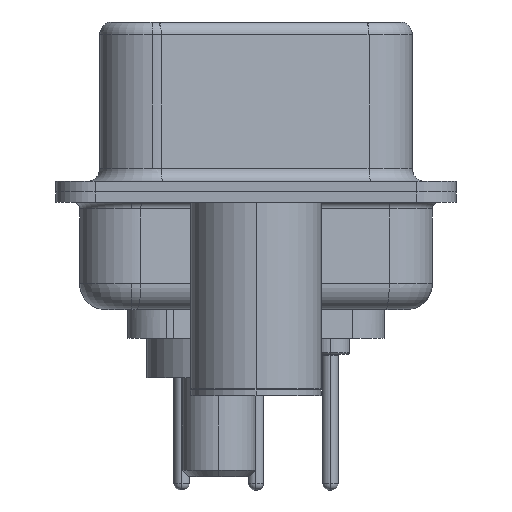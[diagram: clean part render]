
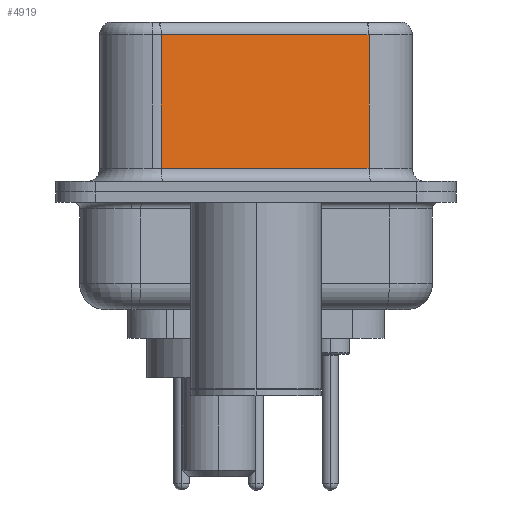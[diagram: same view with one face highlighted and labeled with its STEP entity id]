
A CAD part, left-side view. The second image highlights one B-rep face of the part: STEP entity #4919.
In plain terms, the highlighted planar face has unit normal (-0.985, -0.174, 0).
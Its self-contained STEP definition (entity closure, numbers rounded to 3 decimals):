
#663 = CARTESIAN_POINT ( 'NONE',  ( 5.132, -4.322, 6.52 ) ) ;
#1661 = ORIENTED_EDGE ( 'NONE', *, *, #18239, .T. ) ;
#2152 = CARTESIAN_POINT ( 'NONE',  ( 5.132, -4.322, 0.9 ) ) ;
#4515 = DIRECTION ( 'NONE',  ( 0.174, -0.985, 0. ) ) ;
#4919 = ADVANCED_FACE ( 'NONE', ( #16928 ), #21249, .F. ) ;
#6207 = VECTOR ( 'NONE', #4515, 1000. ) ;
#6247 = LINE ( 'NONE', #15076, #17200 ) ;
#6613 = EDGE_CURVE ( 'NONE', #14384, #29635, #6247, .T. ) ;
#6667 = CARTESIAN_POINT ( 'NONE',  ( 5.132, -4.322, 0.9 ) ) ;
#8347 = DIRECTION ( 'NONE',  ( -0.174, 0.985, 0. ) ) ;
#10439 = CARTESIAN_POINT ( 'NONE',  ( 3.73, 3.628, 6.02 ) ) ;
#14384 = VERTEX_POINT ( 'NONE', #10439 ) ;
#14598 = EDGE_LOOP ( 'NONE', ( #26500, #28176, #25835, #1661 ) ) ;
#15076 = CARTESIAN_POINT ( 'NONE',  ( 3.73, 3.628, 6.52 ) ) ;
#15160 = VECTOR ( 'NONE', #17136, 1000. ) ;
#15279 = CARTESIAN_POINT ( 'NONE',  ( 5.132, -4.322, 6.02 ) ) ;
#16050 = LINE ( 'NONE', #15279, #27094 ) ;
#16928 = FACE_OUTER_BOUND ( 'NONE', #14598, .T. ) ;
#17136 = DIRECTION ( 'NONE',  ( 0., 0., -1. ) ) ;
#17157 = DIRECTION ( 'NONE',  ( 0.985, 0.174, 0. ) ) ;
#17200 = VECTOR ( 'NONE', #29497, 1000. ) ;
#18239 = EDGE_CURVE ( 'NONE', #29635, #24849, #25641, .T. ) ;
#19503 = DIRECTION ( 'NONE',  ( -0.174, 0.985, 0. ) ) ;
#20100 = AXIS2_PLACEMENT_3D ( 'NONE', #20943, #17157, #19503 ) ;
#20943 = CARTESIAN_POINT ( 'NONE',  ( 5.132, -4.322, 6.52 ) ) ;
#21249 = PLANE ( 'NONE',  #20100 ) ;
#22984 = EDGE_CURVE ( 'NONE', #23324, #24849, #27692, .T. ) ;
#23324 = VERTEX_POINT ( 'NONE', #25821 ) ;
#24849 = VERTEX_POINT ( 'NONE', #6667 ) ;
#25641 = LINE ( 'NONE', #2152, #6207 ) ;
#25821 = CARTESIAN_POINT ( 'NONE',  ( 5.132, -4.322, 6.02 ) ) ;
#25835 = ORIENTED_EDGE ( 'NONE', *, *, #6613, .T. ) ;
#26500 = ORIENTED_EDGE ( 'NONE', *, *, #22984, .F. ) ;
#27094 = VECTOR ( 'NONE', #8347, 1000. ) ;
#27159 = EDGE_CURVE ( 'NONE', #23324, #14384, #16050, .T. ) ;
#27692 = LINE ( 'NONE', #663, #15160 ) ;
#28176 = ORIENTED_EDGE ( 'NONE', *, *, #27159, .T. ) ;
#29497 = DIRECTION ( 'NONE',  ( 0., 0., -1. ) ) ;
#29635 = VERTEX_POINT ( 'NONE', #29796 ) ;
#29796 = CARTESIAN_POINT ( 'NONE',  ( 3.73, 3.628, 0.9 ) ) ;
